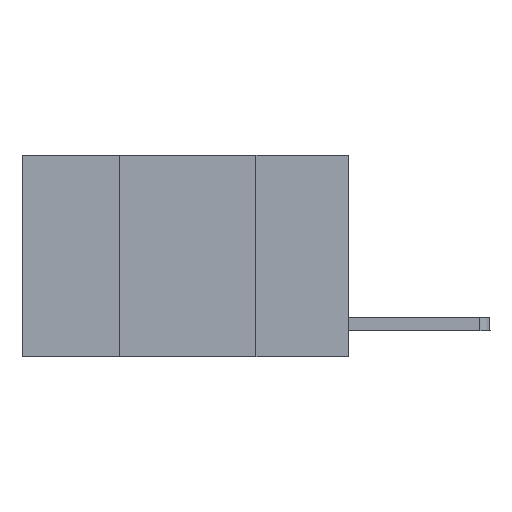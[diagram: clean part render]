
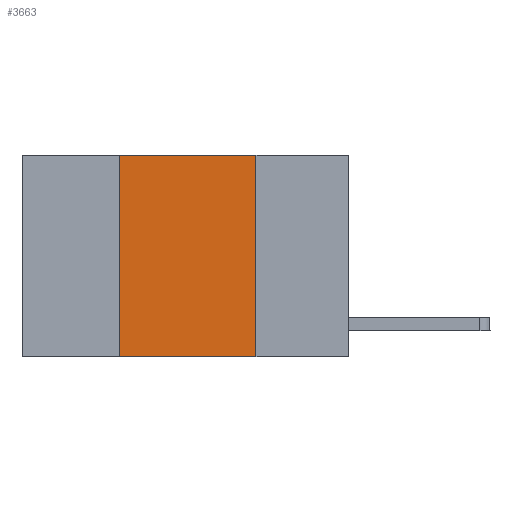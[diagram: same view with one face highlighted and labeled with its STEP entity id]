
A CAD part, left-side view. The second image highlights one B-rep face of the part: STEP entity #3663.
In plain terms, the highlighted planar face has unit normal (-1, 0, 0).
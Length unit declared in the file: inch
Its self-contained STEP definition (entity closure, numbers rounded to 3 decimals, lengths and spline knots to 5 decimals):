
#99 = LINE ( 'NONE', #4375, #5092 ) ;
#282 = VECTOR ( 'NONE', #7288, 39.37008 ) ;
#535 = CARTESIAN_POINT ( 'NONE',  ( 0., 0.6, 0. ) ) ;
#709 = PLANE ( 'NONE',  #11040 ) ;
#1204 = EDGE_CURVE ( 'NONE', #8013, #2604, #99, .T. ) ;
#1219 = CARTESIAN_POINT ( 'NONE',  ( 0., 0.42, 0. ) ) ;
#1256 = ORIENTED_EDGE ( 'NONE', *, *, #3139, .F. ) ;
#1420 = DIRECTION ( 'NONE',  ( 0., 0., -1. ) ) ;
#2078 = LINE ( 'NONE', #1219, #4506 ) ;
#2604 = VERTEX_POINT ( 'NONE', #4276 ) ;
#2749 = VERTEX_POINT ( 'NONE', #5796 ) ;
#2961 = DIRECTION ( 'NONE',  ( 0., 0., 1. ) ) ;
#3139 = EDGE_CURVE ( 'NONE', #7209, #2749, #2078, .T. ) ;
#3214 = DIRECTION ( 'NONE',  ( 1., 0., 0. ) ) ;
#3463 = EDGE_CURVE ( 'NONE', #7209, #2604, #5385, .T. ) ;
#3663 = ADVANCED_FACE ( 'NONE', ( #8189 ), #709, .F. ) ;
#4045 = CARTESIAN_POINT ( 'NONE',  ( 0., 0.42, -0.37 ) ) ;
#4276 = CARTESIAN_POINT ( 'NONE',  ( 0., 0.17, -0.37 ) ) ;
#4375 = CARTESIAN_POINT ( 'NONE',  ( 0., 0.17, 0. ) ) ;
#4506 = VECTOR ( 'NONE', #2961, 39.37008 ) ;
#4832 = CARTESIAN_POINT ( 'NONE',  ( 0., 0.6, 0. ) ) ;
#5092 = VECTOR ( 'NONE', #7817, 39.37008 ) ;
#5385 = LINE ( 'NONE', #8141, #282 ) ;
#5406 = EDGE_LOOP ( 'NONE', ( #10343, #7432, #1256, #7232 ) ) ;
#5796 = CARTESIAN_POINT ( 'NONE',  ( 0., 0.42, 0. ) ) ;
#5914 = CARTESIAN_POINT ( 'NONE',  ( 0., 0.17, 0. ) ) ;
#6632 = LINE ( 'NONE', #4832, #7933 ) ;
#7209 = VERTEX_POINT ( 'NONE', #4045 ) ;
#7232 = ORIENTED_EDGE ( 'NONE', *, *, #3463, .T. ) ;
#7288 = DIRECTION ( 'NONE',  ( 0., -1., 0. ) ) ;
#7432 = ORIENTED_EDGE ( 'NONE', *, *, #8808, .F. ) ;
#7817 = DIRECTION ( 'NONE',  ( 0., 0., -1. ) ) ;
#7933 = VECTOR ( 'NONE', #10073, 39.37008 ) ;
#8013 = VERTEX_POINT ( 'NONE', #5914 ) ;
#8141 = CARTESIAN_POINT ( 'NONE',  ( 0., 0.6, -0.37 ) ) ;
#8189 = FACE_OUTER_BOUND ( 'NONE', #5406, .T. ) ;
#8808 = EDGE_CURVE ( 'NONE', #2749, #8013, #6632, .T. ) ;
#10073 = DIRECTION ( 'NONE',  ( 0., -1., 0. ) ) ;
#10343 = ORIENTED_EDGE ( 'NONE', *, *, #1204, .F. ) ;
#11040 = AXIS2_PLACEMENT_3D ( 'NONE', #535, #3214, #1420 ) ;
